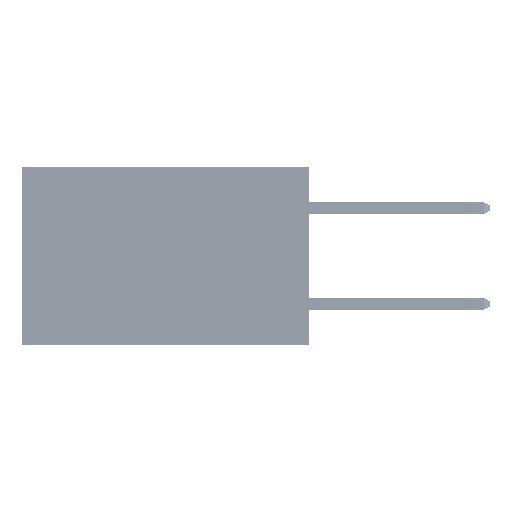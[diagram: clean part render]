
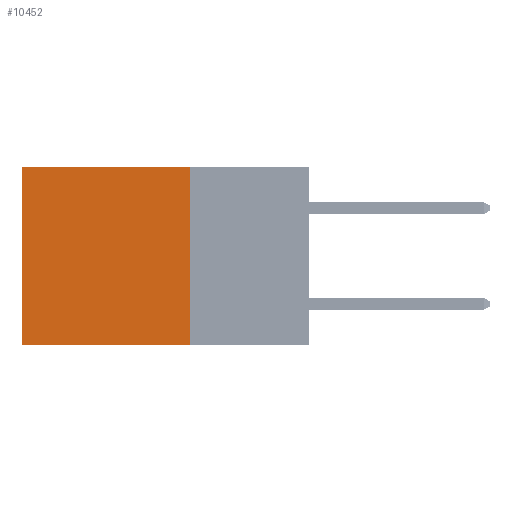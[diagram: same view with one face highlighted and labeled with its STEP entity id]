
A CAD part, left-side view. The second image highlights one B-rep face of the part: STEP entity #10452.
In plain terms, the highlighted planar face has unit normal (-1, 0, 0).
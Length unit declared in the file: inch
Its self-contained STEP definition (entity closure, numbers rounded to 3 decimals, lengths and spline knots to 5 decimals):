
#1193 = ORIENTED_EDGE ( 'NONE', *, *, #27464, .F. ) ;
#1239 = EDGE_LOOP ( 'NONE', ( #12737, #7047, #1193, #44214 ) ) ;
#2679 = CARTESIAN_POINT ( 'NONE',  ( 0.2875, 0.25, 0. ) ) ;
#2850 = PLANE ( 'NONE',  #15416 ) ;
#5499 = CARTESIAN_POINT ( 'NONE',  ( 0.2875, 0.6, 0. ) ) ;
#5817 = VECTOR ( 'NONE', #49266, 39.37008 ) ;
#6882 = CARTESIAN_POINT ( 'NONE',  ( 0.2875, 0.6, -0.37 ) ) ;
#7047 = ORIENTED_EDGE ( 'NONE', *, *, #28048, .F. ) ;
#7319 = CARTESIAN_POINT ( 'NONE',  ( 0.2875, 0.6, 0. ) ) ;
#10452 = ADVANCED_FACE ( 'NONE', ( #19789 ), #2850, .F. ) ;
#11770 = VECTOR ( 'NONE', #47044, 39.37008 ) ;
#12528 = LINE ( 'NONE', #18384, #21508 ) ;
#12737 = ORIENTED_EDGE ( 'NONE', *, *, #16129, .T. ) ;
#14096 = CARTESIAN_POINT ( 'NONE',  ( 0.2875, 0.25, 0. ) ) ;
#15416 = AXIS2_PLACEMENT_3D ( 'NONE', #2679, #44813, #34348 ) ;
#15555 = VERTEX_POINT ( 'NONE', #5499 ) ;
#16129 = EDGE_CURVE ( 'NONE', #15555, #24635, #20754, .T. ) ;
#18384 = CARTESIAN_POINT ( 'NONE',  ( 0.2875, 0.25, 0. ) ) ;
#19703 = LINE ( 'NONE', #41992, #5817 ) ;
#19789 = FACE_OUTER_BOUND ( 'NONE', #1239, .T. ) ;
#20754 = LINE ( 'NONE', #7319, #11770 ) ;
#21508 = VECTOR ( 'NONE', #45322, 39.37008 ) ;
#24635 = VERTEX_POINT ( 'NONE', #6882 ) ;
#24774 = CARTESIAN_POINT ( 'NONE',  ( 0.2875, 0.25, -0.37 ) ) ;
#27464 = EDGE_CURVE ( 'NONE', #47802, #34604, #12528, .T. ) ;
#27625 = EDGE_CURVE ( 'NONE', #47802, #15555, #19703, .T. ) ;
#28048 = EDGE_CURVE ( 'NONE', #34604, #24635, #46177, .T. ) ;
#34348 = DIRECTION ( 'NONE',  ( 0., 0., -1. ) ) ;
#34604 = VERTEX_POINT ( 'NONE', #37931 ) ;
#37931 = CARTESIAN_POINT ( 'NONE',  ( 0.2875, 0.25, -0.37 ) ) ;
#41992 = CARTESIAN_POINT ( 'NONE',  ( 0.2875, 0.25, 0. ) ) ;
#44214 = ORIENTED_EDGE ( 'NONE', *, *, #27625, .T. ) ;
#44308 = DIRECTION ( 'NONE',  ( 0., 1., 0. ) ) ;
#44813 = DIRECTION ( 'NONE',  ( 1., 0., 0. ) ) ;
#45322 = DIRECTION ( 'NONE',  ( 0., 0., -1. ) ) ;
#46177 = LINE ( 'NONE', #24774, #47946 ) ;
#47044 = DIRECTION ( 'NONE',  ( 0., 0., -1. ) ) ;
#47802 = VERTEX_POINT ( 'NONE', #14096 ) ;
#47946 = VECTOR ( 'NONE', #44308, 39.37008 ) ;
#49266 = DIRECTION ( 'NONE',  ( 0., 1., 0. ) ) ;
